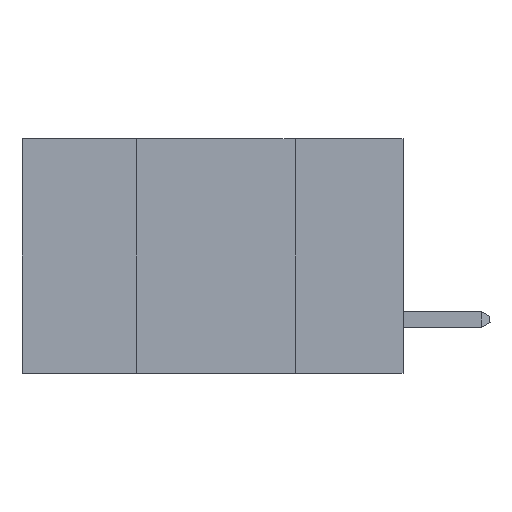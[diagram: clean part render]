
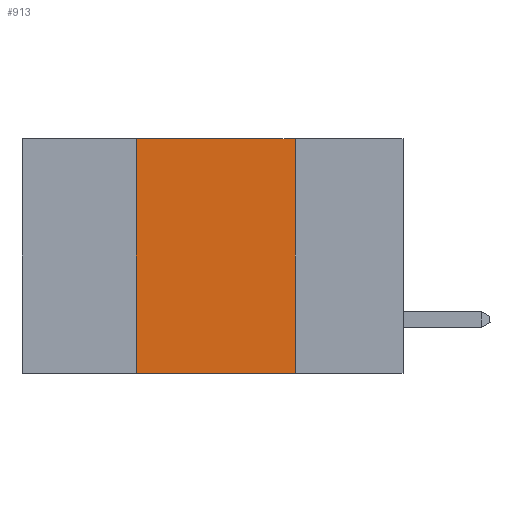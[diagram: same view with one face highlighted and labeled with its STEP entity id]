
A CAD part, left-side view. The second image highlights one B-rep face of the part: STEP entity #913.
In plain terms, the highlighted planar face has unit normal (-1, 0, 0).
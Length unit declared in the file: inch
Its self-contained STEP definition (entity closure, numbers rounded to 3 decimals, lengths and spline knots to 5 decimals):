
#486 = VERTEX_POINT ( 'NONE', #22827 ) ;
#913 = ADVANCED_FACE ( 'NONE', ( #18409 ), #24105, .F. ) ;
#1573 = ORIENTED_EDGE ( 'NONE', *, *, #15219, .F. ) ;
#1834 = CARTESIAN_POINT ( 'NONE',  ( 0., 0.42, -0.37 ) ) ;
#2302 = ORIENTED_EDGE ( 'NONE', *, *, #27575, .T. ) ;
#3380 = LINE ( 'NONE', #20161, #8832 ) ;
#3870 = VERTEX_POINT ( 'NONE', #1834 ) ;
#6799 = VERTEX_POINT ( 'NONE', #15188 ) ;
#6821 = LINE ( 'NONE', #9914, #15976 ) ;
#7528 = CARTESIAN_POINT ( 'NONE',  ( 0., 0.6, -0.37 ) ) ;
#8832 = VECTOR ( 'NONE', #24600, 39.37008 ) ;
#9078 = ORIENTED_EDGE ( 'NONE', *, *, #18611, .F. ) ;
#9914 = CARTESIAN_POINT ( 'NONE',  ( 0., 0.17, 0. ) ) ;
#10244 = EDGE_LOOP ( 'NONE', ( #9078, #22127, #1573, #2302 ) ) ;
#10535 = CARTESIAN_POINT ( 'NONE',  ( 0., 0.42, 0. ) ) ;
#11078 = LINE ( 'NONE', #10535, #14492 ) ;
#11146 = CARTESIAN_POINT ( 'NONE',  ( 0., 0.6, 0. ) ) ;
#14040 = DIRECTION ( 'NONE',  ( 0., -1., 0. ) ) ;
#14492 = VECTOR ( 'NONE', #21294, 39.37008 ) ;
#15188 = CARTESIAN_POINT ( 'NONE',  ( 0., 0.42, 0. ) ) ;
#15219 = EDGE_CURVE ( 'NONE', #3870, #6799, #11078, .T. ) ;
#15567 = LINE ( 'NONE', #7528, #22991 ) ;
#15976 = VECTOR ( 'NONE', #23326, 39.37008 ) ;
#18409 = FACE_OUTER_BOUND ( 'NONE', #10244, .T. ) ;
#18611 = EDGE_CURVE ( 'NONE', #486, #26475, #6821, .T. ) ;
#20161 = CARTESIAN_POINT ( 'NONE',  ( 0., 0.6, 0. ) ) ;
#21294 = DIRECTION ( 'NONE',  ( 0., 0., 1. ) ) ;
#22012 = DIRECTION ( 'NONE',  ( 1., 0., 0. ) ) ;
#22127 = ORIENTED_EDGE ( 'NONE', *, *, #26437, .F. ) ;
#22827 = CARTESIAN_POINT ( 'NONE',  ( 0., 0.17, 0. ) ) ;
#22991 = VECTOR ( 'NONE', #14040, 39.37008 ) ;
#23326 = DIRECTION ( 'NONE',  ( 0., 0., -1. ) ) ;
#24105 = PLANE ( 'NONE',  #26988 ) ;
#24600 = DIRECTION ( 'NONE',  ( 0., -1., 0. ) ) ;
#26299 = DIRECTION ( 'NONE',  ( 0., 0., -1. ) ) ;
#26437 = EDGE_CURVE ( 'NONE', #6799, #486, #3380, .T. ) ;
#26475 = VERTEX_POINT ( 'NONE', #26623 ) ;
#26623 = CARTESIAN_POINT ( 'NONE',  ( 0., 0.17, -0.37 ) ) ;
#26988 = AXIS2_PLACEMENT_3D ( 'NONE', #11146, #22012, #26299 ) ;
#27575 = EDGE_CURVE ( 'NONE', #3870, #26475, #15567, .T. ) ;
